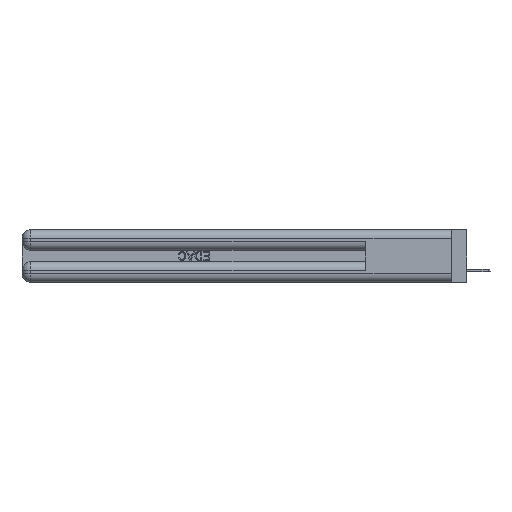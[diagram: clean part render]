
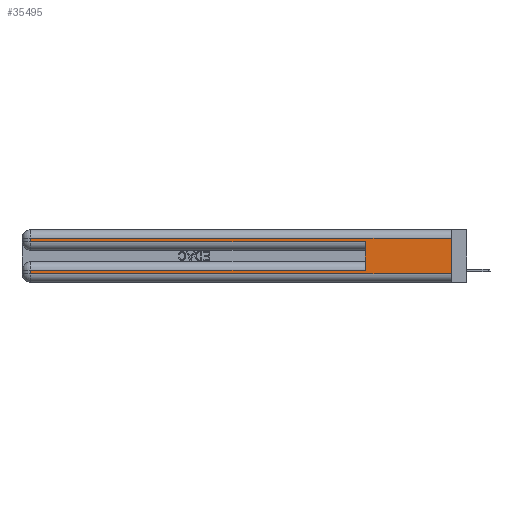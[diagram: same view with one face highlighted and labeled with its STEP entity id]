
A CAD part, left-side view. The second image highlights one B-rep face of the part: STEP entity #35495.
In plain terms, the highlighted planar face has unit normal (-1, 0, 0).
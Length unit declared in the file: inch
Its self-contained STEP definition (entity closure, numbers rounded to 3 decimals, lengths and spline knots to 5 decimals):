
#223 = CARTESIAN_POINT ( 'NONE',  ( 0., 0., 0.285 ) ) ;
#381 = CARTESIAN_POINT ( 'NONE',  ( 0., 2.94, 0.085 ) ) ;
#614 = ORIENTED_EDGE ( 'NONE', *, *, #10982, .T. ) ;
#1441 = ORIENTED_EDGE ( 'NONE', *, *, #3932, .F. ) ;
#1590 = CARTESIAN_POINT ( 'NONE',  ( 0., 0., 0.31 ) ) ;
#2123 = LINE ( 'NONE', #25085, #21978 ) ;
#2686 = EDGE_CURVE ( 'NONE', #38724, #21392, #18399, .T. ) ;
#3581 = CARTESIAN_POINT ( 'NONE',  ( 0., 0., 0.37 ) ) ;
#3829 = DIRECTION ( 'NONE',  ( 0., 0., -1. ) ) ;
#3932 = EDGE_CURVE ( 'NONE', #7380, #26691, #19808, .T. ) ;
#4227 = EDGE_CURVE ( 'NONE', #7380, #4953, #29448, .T. ) ;
#4953 = VERTEX_POINT ( 'NONE', #20604 ) ;
#5589 = CARTESIAN_POINT ( 'NONE',  ( 0., 0.6, 0.285 ) ) ;
#7380 = VERTEX_POINT ( 'NONE', #37415 ) ;
#7656 = ORIENTED_EDGE ( 'NONE', *, *, #4227, .T. ) ;
#7729 = CARTESIAN_POINT ( 'NONE',  ( 0., 0.6, 0.085 ) ) ;
#7878 = FACE_OUTER_BOUND ( 'NONE', #26476, .T. ) ;
#8143 = LINE ( 'NONE', #223, #22745 ) ;
#8821 = ORIENTED_EDGE ( 'NONE', *, *, #15578, .T. ) ;
#9306 = CARTESIAN_POINT ( 'NONE',  ( 0., 2.94, 0.37 ) ) ;
#10982 = EDGE_CURVE ( 'NONE', #21392, #27242, #12038, .T. ) ;
#11435 = DIRECTION ( 'NONE',  ( 0., 0., -1. ) ) ;
#11831 = PLANE ( 'NONE',  #31257 ) ;
#12038 = LINE ( 'NONE', #28262, #22756 ) ;
#13187 = CARTESIAN_POINT ( 'NONE',  ( 0., 2.94, 0.285 ) ) ;
#13800 = DIRECTION ( 'NONE',  ( 0., 0., 1. ) ) ;
#13980 = CARTESIAN_POINT ( 'NONE',  ( 0., 2.94, 0.06 ) ) ;
#14753 = ORIENTED_EDGE ( 'NONE', *, *, #15452, .T. ) ;
#15452 = EDGE_CURVE ( 'NONE', #4953, #26914, #17600, .T. ) ;
#15578 = EDGE_CURVE ( 'NONE', #27242, #26691, #2123, .T. ) ;
#15741 = DIRECTION ( 'NONE',  ( 0., -1., 0. ) ) ;
#16593 = DIRECTION ( 'NONE',  ( 0., 1., 0. ) ) ;
#17600 = LINE ( 'NONE', #9306, #23456 ) ;
#18109 = DIRECTION ( 'NONE',  ( 0., 1., 0. ) ) ;
#18399 = LINE ( 'NONE', #20428, #23738 ) ;
#19314 = LINE ( 'NONE', #32133, #20772 ) ;
#19808 = LINE ( 'NONE', #3581, #25154 ) ;
#20428 = CARTESIAN_POINT ( 'NONE',  ( 0., 0., 0.085 ) ) ;
#20604 = CARTESIAN_POINT ( 'NONE',  ( 0., 2.94, 0.31 ) ) ;
#20772 = VECTOR ( 'NONE', #13800, 39.37008 ) ;
#21215 = VECTOR ( 'NONE', #16593, 39.37008 ) ;
#21392 = VERTEX_POINT ( 'NONE', #381 ) ;
#21889 = ORIENTED_EDGE ( 'NONE', *, *, #37965, .T. ) ;
#21978 = VECTOR ( 'NONE', #28050, 39.37008 ) ;
#22745 = VECTOR ( 'NONE', #15741, 39.37008 ) ;
#22756 = VECTOR ( 'NONE', #28668, 39.37008 ) ;
#23456 = VECTOR ( 'NONE', #25215, 39.37008 ) ;
#23738 = VECTOR ( 'NONE', #18109, 39.37008 ) ;
#23972 = CARTESIAN_POINT ( 'NONE',  ( 0., 0., 0.06 ) ) ;
#25085 = CARTESIAN_POINT ( 'NONE',  ( 0., 0., 0.06 ) ) ;
#25154 = VECTOR ( 'NONE', #3829, 39.37008 ) ;
#25215 = DIRECTION ( 'NONE',  ( 0., 0., -1. ) ) ;
#26476 = EDGE_LOOP ( 'NONE', ( #1441, #7656, #14753, #21889, #39346, #26687, #614, #8821 ) ) ;
#26687 = ORIENTED_EDGE ( 'NONE', *, *, #2686, .T. ) ;
#26691 = VERTEX_POINT ( 'NONE', #23972 ) ;
#26914 = VERTEX_POINT ( 'NONE', #13187 ) ;
#27242 = VERTEX_POINT ( 'NONE', #13980 ) ;
#28050 = DIRECTION ( 'NONE',  ( 0., -1., 0. ) ) ;
#28262 = CARTESIAN_POINT ( 'NONE',  ( 0., 2.94, 0.37 ) ) ;
#28668 = DIRECTION ( 'NONE',  ( 0., 0., -1. ) ) ;
#29076 = VERTEX_POINT ( 'NONE', #5589 ) ;
#29448 = LINE ( 'NONE', #1590, #21215 ) ;
#30435 = CARTESIAN_POINT ( 'NONE',  ( 0., 0., 0.37 ) ) ;
#31257 = AXIS2_PLACEMENT_3D ( 'NONE', #30435, #33678, #11435 ) ;
#32133 = CARTESIAN_POINT ( 'NONE',  ( 0., 0.6, 0.145 ) ) ;
#33678 = DIRECTION ( 'NONE',  ( 1., 0., 0. ) ) ;
#35495 = ADVANCED_FACE ( 'NONE', ( #7878 ), #11831, .F. ) ;
#37415 = CARTESIAN_POINT ( 'NONE',  ( 0., 0., 0.31 ) ) ;
#37965 = EDGE_CURVE ( 'NONE', #26914, #29076, #8143, .T. ) ;
#38285 = EDGE_CURVE ( 'NONE', #38724, #29076, #19314, .T. ) ;
#38724 = VERTEX_POINT ( 'NONE', #7729 ) ;
#39346 = ORIENTED_EDGE ( 'NONE', *, *, #38285, .F. ) ;
